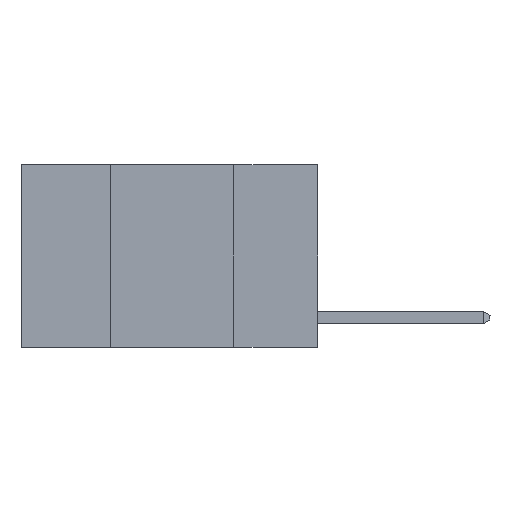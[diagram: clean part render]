
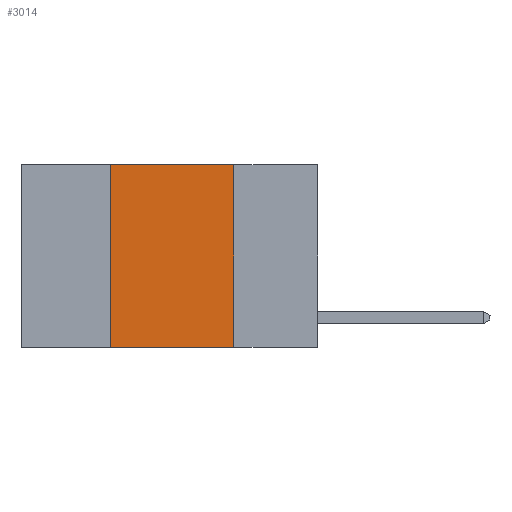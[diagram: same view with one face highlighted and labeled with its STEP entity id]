
A CAD part, left-side view. The second image highlights one B-rep face of the part: STEP entity #3014.
In plain terms, the highlighted planar face has unit normal (-1, 0, 0).
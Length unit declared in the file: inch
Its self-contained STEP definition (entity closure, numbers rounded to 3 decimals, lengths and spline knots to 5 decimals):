
#83 = CARTESIAN_POINT ( 'NONE',  ( 0., 0.42, 0. ) ) ;
#165 = LINE ( 'NONE', #10029, #2556 ) ;
#475 = EDGE_CURVE ( 'NONE', #8464, #6499, #4904, .T. ) ;
#621 = EDGE_CURVE ( 'NONE', #3666, #2694, #5372, .T. ) ;
#795 = EDGE_CURVE ( 'NONE', #8464, #3666, #11223, .T. ) ;
#1679 = PLANE ( 'NONE',  #7671 ) ;
#2044 = ORIENTED_EDGE ( 'NONE', *, *, #7393, .F. ) ;
#2077 = FACE_OUTER_BOUND ( 'NONE', #3743, .T. ) ;
#2218 = CARTESIAN_POINT ( 'NONE',  ( 0., 0.42, -0.37 ) ) ;
#2279 = VECTOR ( 'NONE', #11539, 39.37008 ) ;
#2328 = ORIENTED_EDGE ( 'NONE', *, *, #795, .F. ) ;
#2556 = VECTOR ( 'NONE', #10969, 39.37008 ) ;
#2694 = VERTEX_POINT ( 'NONE', #10589 ) ;
#3014 = ADVANCED_FACE ( 'NONE', ( #2077 ), #1679, .F. ) ;
#3666 = VERTEX_POINT ( 'NONE', #83 ) ;
#3743 = EDGE_LOOP ( 'NONE', ( #2044, #12277, #2328, #10101 ) ) ;
#3782 = DIRECTION ( 'NONE',  ( 1., 0., 0. ) ) ;
#3962 = DIRECTION ( 'NONE',  ( 0., 0., 1. ) ) ;
#4904 = LINE ( 'NONE', #5243, #2279 ) ;
#5023 = CARTESIAN_POINT ( 'NONE',  ( 0., 0.6, 0. ) ) ;
#5243 = CARTESIAN_POINT ( 'NONE',  ( 0., 0.6, -0.37 ) ) ;
#5372 = LINE ( 'NONE', #12011, #10488 ) ;
#6499 = VERTEX_POINT ( 'NONE', #10538 ) ;
#7393 = EDGE_CURVE ( 'NONE', #2694, #6499, #165, .T. ) ;
#7671 = AXIS2_PLACEMENT_3D ( 'NONE', #5023, #3782, #9223 ) ;
#7863 = DIRECTION ( 'NONE',  ( 0., -1., 0. ) ) ;
#8464 = VERTEX_POINT ( 'NONE', #2218 ) ;
#9105 = CARTESIAN_POINT ( 'NONE',  ( 0., 0.42, 0. ) ) ;
#9223 = DIRECTION ( 'NONE',  ( 0., 0., -1. ) ) ;
#10029 = CARTESIAN_POINT ( 'NONE',  ( 0., 0.17, 0. ) ) ;
#10101 = ORIENTED_EDGE ( 'NONE', *, *, #475, .T. ) ;
#10488 = VECTOR ( 'NONE', #7863, 39.37008 ) ;
#10538 = CARTESIAN_POINT ( 'NONE',  ( 0., 0.17, -0.37 ) ) ;
#10589 = CARTESIAN_POINT ( 'NONE',  ( 0., 0.17, 0. ) ) ;
#10639 = VECTOR ( 'NONE', #3962, 39.37008 ) ;
#10969 = DIRECTION ( 'NONE',  ( 0., 0., -1. ) ) ;
#11223 = LINE ( 'NONE', #9105, #10639 ) ;
#11539 = DIRECTION ( 'NONE',  ( 0., -1., 0. ) ) ;
#12011 = CARTESIAN_POINT ( 'NONE',  ( 0., 0.6, 0. ) ) ;
#12277 = ORIENTED_EDGE ( 'NONE', *, *, #621, .F. ) ;
